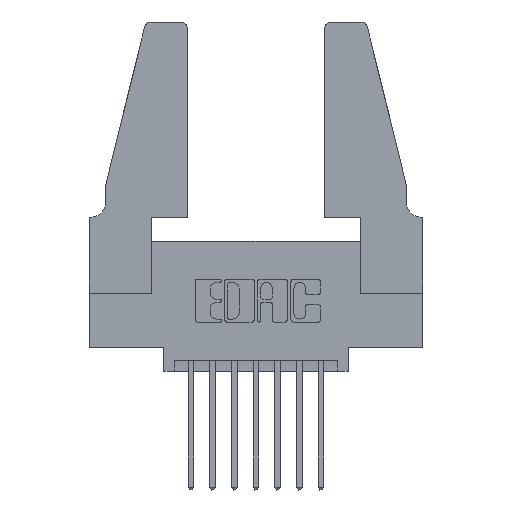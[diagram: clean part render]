
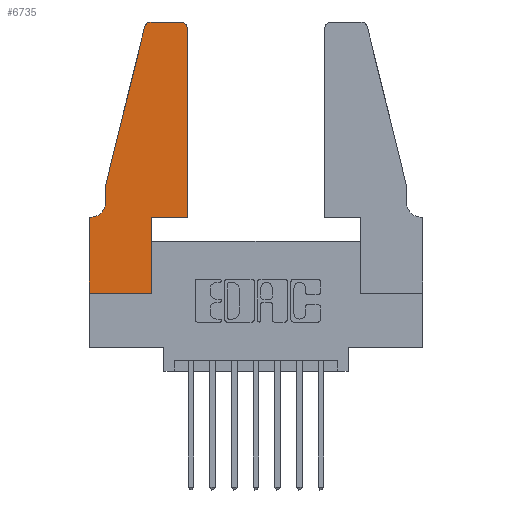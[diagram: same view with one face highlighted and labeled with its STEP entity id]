
A CAD part, top view. The second image highlights one B-rep face of the part: STEP entity #6735.
In plain terms, the highlighted planar face has unit normal (0, 0, 1).
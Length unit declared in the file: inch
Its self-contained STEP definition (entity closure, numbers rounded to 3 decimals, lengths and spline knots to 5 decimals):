
#12 = DIRECTION ( 'NONE',  ( 0., -1., 0. ) ) ;
#252 = CARTESIAN_POINT ( 'NONE',  ( 0.4505, 0.35, 0.37 ) ) ;
#331 = VERTEX_POINT ( 'NONE', #3127 ) ;
#380 = CARTESIAN_POINT ( 'NONE',  ( 0.2865, 0.35, 0.37 ) ) ;
#688 = LINE ( 'NONE', #7775, #2178 ) ;
#717 = CARTESIAN_POINT ( 'NONE',  ( 0.4505, 0.35, 0.37 ) ) ;
#894 = EDGE_CURVE ( 'NONE', #9570, #12159, #7222, .T. ) ;
#900 = ORIENTED_EDGE ( 'NONE', *, *, #2320, .T. ) ;
#1276 = LINE ( 'NONE', #7959, #10065 ) ;
#1292 = ORIENTED_EDGE ( 'NONE', *, *, #4139, .T. ) ;
#1299 = CARTESIAN_POINT ( 'NONE',  ( 0., 0., 0.37 ) ) ;
#1702 = CARTESIAN_POINT ( 'NONE',  ( 0.284, 1.25, 0.37 ) ) ;
#1778 = EDGE_CURVE ( 'NONE', #12159, #4316, #1276, .T. ) ;
#1830 = CARTESIAN_POINT ( 'NONE',  ( 0.284, 1.22, 0.37 ) ) ;
#1932 = AXIS2_PLACEMENT_3D ( 'NONE', #4016, #3079, #4882 ) ;
#2131 = CARTESIAN_POINT ( 'NONE',  ( 0.4205, 1.22, 0.37 ) ) ;
#2178 = VECTOR ( 'NONE', #8446, 39.37008 ) ;
#2320 = EDGE_CURVE ( 'NONE', #11454, #2611, #688, .T. ) ;
#2400 = DIRECTION ( 'NONE',  ( 1., 0., 0. ) ) ;
#2473 = CARTESIAN_POINT ( 'NONE',  ( 0.0755, 0.5, 0.37 ) ) ;
#2495 = LINE ( 'NONE', #2604, #5408 ) ;
#2512 = DIRECTION ( 'NONE',  ( 1., 0., 0. ) ) ;
#2604 = CARTESIAN_POINT ( 'NONE',  ( 0.4505, 0.35, 0.37 ) ) ;
#2611 = VERTEX_POINT ( 'NONE', #380 ) ;
#3030 = CARTESIAN_POINT ( 'NONE',  ( 0.0755, 0.5, 0.37 ) ) ;
#3056 = ORIENTED_EDGE ( 'NONE', *, *, #7822, .T. ) ;
#3060 = VECTOR ( 'NONE', #4455, 39.37008 ) ;
#3079 = DIRECTION ( 'NONE',  ( 0., 0., 1. ) ) ;
#3115 = AXIS2_PLACEMENT_3D ( 'NONE', #1830, #4196, #4971 ) ;
#3127 = CARTESIAN_POINT ( 'NONE',  ( 0., 0., 0.37 ) ) ;
#3242 = CARTESIAN_POINT ( 'NONE',  ( 0.2865, 0., 0.37 ) ) ;
#3711 = LINE ( 'NONE', #5380, #3060 ) ;
#3837 = CARTESIAN_POINT ( 'NONE',  ( 0.25487, 1.22718, 0.37 ) ) ;
#3881 = CARTESIAN_POINT ( 'NONE',  ( 0., 0., 0.37 ) ) ;
#4003 = ORIENTED_EDGE ( 'NONE', *, *, #6230, .T. ) ;
#4016 = CARTESIAN_POINT ( 'NONE',  ( 0., 0.35, 0.37 ) ) ;
#4034 = ORIENTED_EDGE ( 'NONE', *, *, #11572, .T. ) ;
#4056 = DIRECTION ( 'NONE',  ( 0., 0., 1. ) ) ;
#4139 = EDGE_CURVE ( 'NONE', #4316, #331, #12426, .T. ) ;
#4143 = DIRECTION ( 'NONE',  ( -1., 0., 0. ) ) ;
#4196 = DIRECTION ( 'NONE',  ( 0., 0., 1. ) ) ;
#4269 = VERTEX_POINT ( 'NONE', #6105 ) ;
#4316 = VERTEX_POINT ( 'NONE', #11137 ) ;
#4439 = VECTOR ( 'NONE', #12, 39.37008 ) ;
#4455 = DIRECTION ( 'NONE',  ( -1., 0., 0. ) ) ;
#4882 = DIRECTION ( 'NONE',  ( 1., 0., 0. ) ) ;
#4971 = DIRECTION ( 'NONE',  ( 1., 0., 0. ) ) ;
#5380 = CARTESIAN_POINT ( 'NONE',  ( 0.2605, 1.25, 0.37 ) ) ;
#5408 = VECTOR ( 'NONE', #2512, 39.37008 ) ;
#5565 = VECTOR ( 'NONE', #2400, 39.37008 ) ;
#5747 = ORIENTED_EDGE ( 'NONE', *, *, #1778, .T. ) ;
#5991 = DIRECTION ( 'NONE',  ( 1., 0., 0. ) ) ;
#6105 = CARTESIAN_POINT ( 'NONE',  ( 0.4505, 1.22, 0.37 ) ) ;
#6123 = DIRECTION ( 'NONE',  ( -1., 0., 0. ) ) ;
#6167 = DIRECTION ( 'NONE',  ( 0., 0., -1. ) ) ;
#6169 = CIRCLE ( 'NONE', #6207, 0.03 ) ;
#6207 = AXIS2_PLACEMENT_3D ( 'NONE', #2131, #4056, #5991 ) ;
#6230 = EDGE_CURVE ( 'NONE', #4269, #12364, #6169, .T. ) ;
#6735 = ADVANCED_FACE ( 'NONE', ( #9899 ), #6989, .T. ) ;
#6857 = DIRECTION ( 'NONE',  ( 0., 1., 0. ) ) ;
#6989 = PLANE ( 'NONE',  #1932 ) ;
#7222 = CIRCLE ( 'NONE', #11364, 0.07 ) ;
#7483 = VECTOR ( 'NONE', #7850, 39.37008 ) ;
#7775 = CARTESIAN_POINT ( 'NONE',  ( 0.2865, 0.35, 0.37 ) ) ;
#7822 = EDGE_CURVE ( 'NONE', #11843, #9570, #10510, .T. ) ;
#7850 = DIRECTION ( 'NONE',  ( 0., -1., 0. ) ) ;
#7917 = LINE ( 'NONE', #8637, #12123 ) ;
#7947 = EDGE_CURVE ( 'NONE', #9732, #11843, #7917, .T. ) ;
#7959 = CARTESIAN_POINT ( 'NONE',  ( 0.0755, 0.35, 0.37 ) ) ;
#8068 = ORIENTED_EDGE ( 'NONE', *, *, #11723, .T. ) ;
#8233 = VERTEX_POINT ( 'NONE', #1702 ) ;
#8446 = DIRECTION ( 'NONE',  ( 0., 1., 0. ) ) ;
#8454 = VECTOR ( 'NONE', #6857, 39.37008 ) ;
#8511 = EDGE_CURVE ( 'NONE', #8233, #9732, #11791, .T. ) ;
#8558 = DIRECTION ( 'NONE',  ( -0.239, -0.971, 0. ) ) ;
#8637 = CARTESIAN_POINT ( 'NONE',  ( 0.0755, 0.5, 0.37 ) ) ;
#9034 = CARTESIAN_POINT ( 'NONE',  ( 0.4205, 1.25, 0.37 ) ) ;
#9370 = LINE ( 'NONE', #717, #8454 ) ;
#9570 = VERTEX_POINT ( 'NONE', #10150 ) ;
#9732 = VERTEX_POINT ( 'NONE', #3837 ) ;
#9869 = ORIENTED_EDGE ( 'NONE', *, *, #12510, .T. ) ;
#9899 = FACE_OUTER_BOUND ( 'NONE', #9912, .T. ) ;
#9912 = EDGE_LOOP ( 'NONE', ( #9869, #11410, #11104, #3056, #12086, #5747, #1292, #4034, #900, #8068, #10224, #4003 ) ) ;
#10065 = VECTOR ( 'NONE', #4143, 39.37008 ) ;
#10150 = CARTESIAN_POINT ( 'NONE',  ( 0.0755, 0.42, 0.37 ) ) ;
#10163 = CARTESIAN_POINT ( 'NONE',  ( 0.0055, 0.42, 0.37 ) ) ;
#10224 = ORIENTED_EDGE ( 'NONE', *, *, #10891, .T. ) ;
#10510 = LINE ( 'NONE', #3030, #7483 ) ;
#10891 = EDGE_CURVE ( 'NONE', #11909, #4269, #9370, .T. ) ;
#11104 = ORIENTED_EDGE ( 'NONE', *, *, #7947, .T. ) ;
#11137 = CARTESIAN_POINT ( 'NONE',  ( 0., 0.35, 0.37 ) ) ;
#11286 = CARTESIAN_POINT ( 'NONE',  ( 0.0055, 0.35, 0.37 ) ) ;
#11364 = AXIS2_PLACEMENT_3D ( 'NONE', #10163, #6167, #6123 ) ;
#11410 = ORIENTED_EDGE ( 'NONE', *, *, #8511, .T. ) ;
#11454 = VERTEX_POINT ( 'NONE', #3242 ) ;
#11572 = EDGE_CURVE ( 'NONE', #331, #11454, #12041, .T. ) ;
#11723 = EDGE_CURVE ( 'NONE', #2611, #11909, #2495, .T. ) ;
#11791 = CIRCLE ( 'NONE', #3115, 0.03 ) ;
#11843 = VERTEX_POINT ( 'NONE', #2473 ) ;
#11909 = VERTEX_POINT ( 'NONE', #252 ) ;
#12041 = LINE ( 'NONE', #1299, #5565 ) ;
#12086 = ORIENTED_EDGE ( 'NONE', *, *, #894, .T. ) ;
#12123 = VECTOR ( 'NONE', #8558, 39.37008 ) ;
#12159 = VERTEX_POINT ( 'NONE', #11286 ) ;
#12364 = VERTEX_POINT ( 'NONE', #9034 ) ;
#12426 = LINE ( 'NONE', #3881, #4439 ) ;
#12510 = EDGE_CURVE ( 'NONE', #12364, #8233, #3711, .T. ) ;
